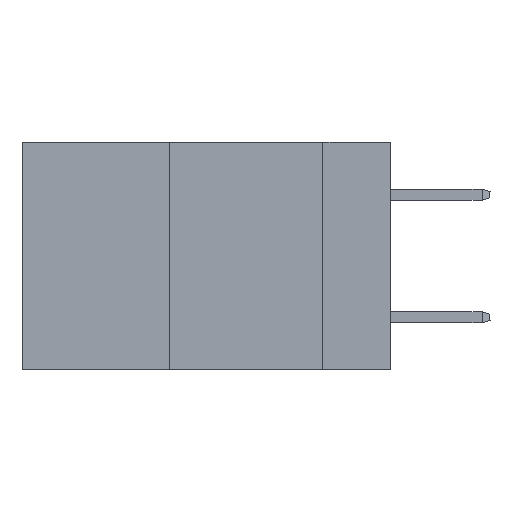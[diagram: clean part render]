
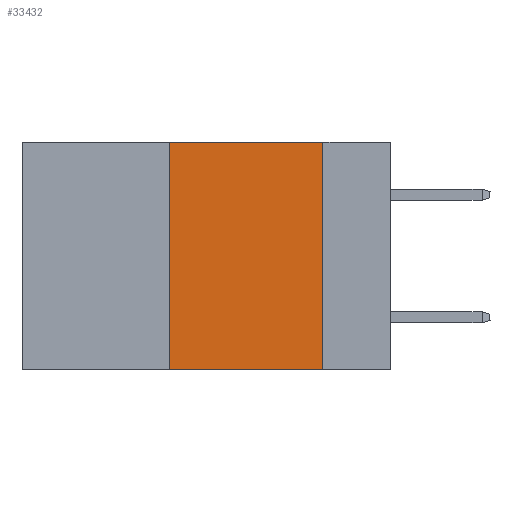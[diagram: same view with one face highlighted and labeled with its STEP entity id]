
A CAD part, left-side view. The second image highlights one B-rep face of the part: STEP entity #33432.
In plain terms, the highlighted planar face has unit normal (-1, 0, 0).
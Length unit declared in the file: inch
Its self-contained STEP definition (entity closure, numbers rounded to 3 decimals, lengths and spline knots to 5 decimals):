
#2369 = ORIENTED_EDGE ( 'NONE', *, *, #31894, .F. ) ;
#3071 = VERTEX_POINT ( 'NONE', #33134 ) ;
#5325 = DIRECTION ( 'NONE',  ( 0., 0., 1. ) ) ;
#6203 = PLANE ( 'NONE',  #6535 ) ;
#6535 = AXIS2_PLACEMENT_3D ( 'NONE', #26621, #9121, #29540 ) ;
#7068 = CARTESIAN_POINT ( 'NONE',  ( 0., 0.36, -0.37 ) ) ;
#7281 = ORIENTED_EDGE ( 'NONE', *, *, #24823, .T. ) ;
#7920 = CARTESIAN_POINT ( 'NONE',  ( 0., 0.6, -0.37 ) ) ;
#8014 = CARTESIAN_POINT ( 'NONE',  ( 0., 0.36, 0. ) ) ;
#8246 = LINE ( 'NONE', #37330, #9589 ) ;
#8846 = DIRECTION ( 'NONE',  ( 0., 0., -1. ) ) ;
#8955 = VECTOR ( 'NONE', #22616, 39.37008 ) ;
#9121 = DIRECTION ( 'NONE',  ( 1., 0., 0. ) ) ;
#9589 = VECTOR ( 'NONE', #37220, 39.37008 ) ;
#10432 = EDGE_CURVE ( 'NONE', #19980, #19731, #31876, .T. ) ;
#11265 = CARTESIAN_POINT ( 'NONE',  ( 0., 0.11, 0. ) ) ;
#16722 = LINE ( 'NONE', #7920, #8955 ) ;
#17274 = VECTOR ( 'NONE', #5325, 39.37008 ) ;
#19731 = VERTEX_POINT ( 'NONE', #8014 ) ;
#19980 = VERTEX_POINT ( 'NONE', #7068 ) ;
#22616 = DIRECTION ( 'NONE',  ( 0., -1., 0. ) ) ;
#23021 = LINE ( 'NONE', #11265, #23076 ) ;
#23076 = VECTOR ( 'NONE', #8846, 39.37008 ) ;
#23473 = VERTEX_POINT ( 'NONE', #34753 ) ;
#23544 = ORIENTED_EDGE ( 'NONE', *, *, #10432, .F. ) ;
#24312 = FACE_OUTER_BOUND ( 'NONE', #36338, .T. ) ;
#24823 = EDGE_CURVE ( 'NONE', #19980, #23473, #16722, .T. ) ;
#26621 = CARTESIAN_POINT ( 'NONE',  ( 0., 0.6, 0. ) ) ;
#29540 = DIRECTION ( 'NONE',  ( 0., 0., -1. ) ) ;
#30952 = ORIENTED_EDGE ( 'NONE', *, *, #36977, .F. ) ;
#31876 = LINE ( 'NONE', #37408, #17274 ) ;
#31894 = EDGE_CURVE ( 'NONE', #3071, #23473, #23021, .T. ) ;
#33134 = CARTESIAN_POINT ( 'NONE',  ( 0., 0.11, 0. ) ) ;
#33432 = ADVANCED_FACE ( 'NONE', ( #24312 ), #6203, .F. ) ;
#34753 = CARTESIAN_POINT ( 'NONE',  ( 0., 0.11, -0.37 ) ) ;
#36338 = EDGE_LOOP ( 'NONE', ( #2369, #30952, #23544, #7281 ) ) ;
#36977 = EDGE_CURVE ( 'NONE', #19731, #3071, #8246, .T. ) ;
#37220 = DIRECTION ( 'NONE',  ( 0., -1., 0. ) ) ;
#37330 = CARTESIAN_POINT ( 'NONE',  ( 0., 0.6, 0. ) ) ;
#37408 = CARTESIAN_POINT ( 'NONE',  ( 0., 0.36, 0. ) ) ;
